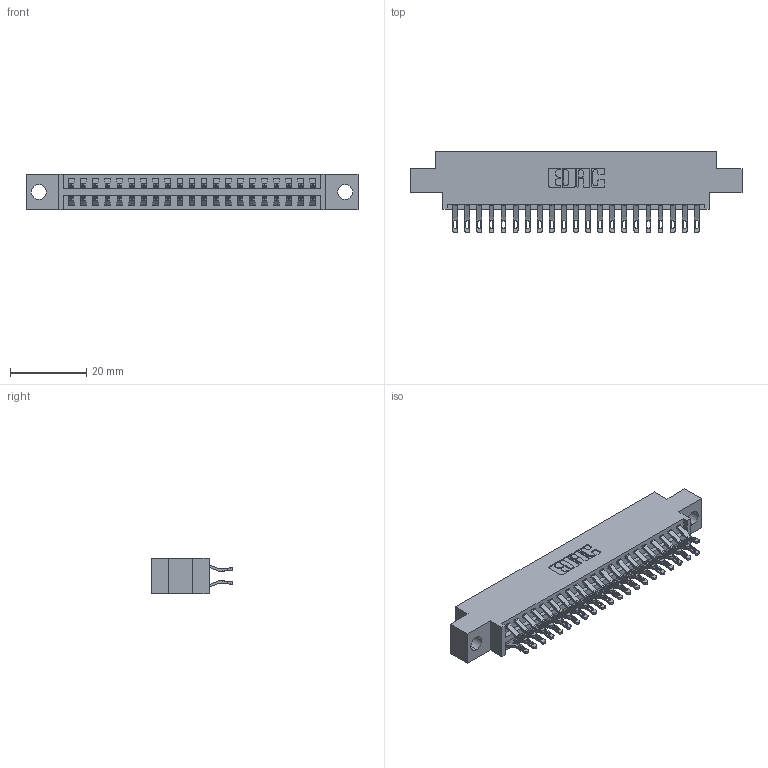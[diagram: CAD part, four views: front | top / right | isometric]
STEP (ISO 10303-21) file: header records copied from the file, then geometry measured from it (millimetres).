
FILE_DESCRIPTION (( 'STEP AP203' ), '1' );
FILE_NAME ('346-042-555-804.STEP', '2022-05-20T04:59:33', ( '' ), ( '' ), 'SwSTEP 2.0', 'SolidWorks 2020', '' );
FILE_SCHEMA (( 'CONFIG_CONTROL_DESIGN' ));
Length unit declared in the file: inch
Products named in the file (3): 346-042-555-804; 346 Part_0.170 Offset - 0.156 Dia-TH; 345-292-001_555 Tail
Assembly tree (43 placements, depth 2):
  346-042-555-804
    346 Part_0.170 Offset - 0.156 Dia-TH
    345-292-001_555 Tail  x42
Bounding box: 87.25 x 21.46 x 9.4 mm (x, y, z)
Volume: 8206 mm3; surface area: 11411.4 mm2
Topology: 43 solids, 43 shells, 2576 faces, 8063 edges, 5374 vertices
Faces by surface type: plane 1480, cylinder 1096
Entity records: 17409 total; most frequent: CARTESIAN_POINT 2940, ORIENTED_EDGE 2842, DIRECTION 2609, EDGE_CURVE 1421, LINE 1185, VECTOR 1185, VERTEX_POINT 946, AXIS2_PLACEMENT_3D 712
